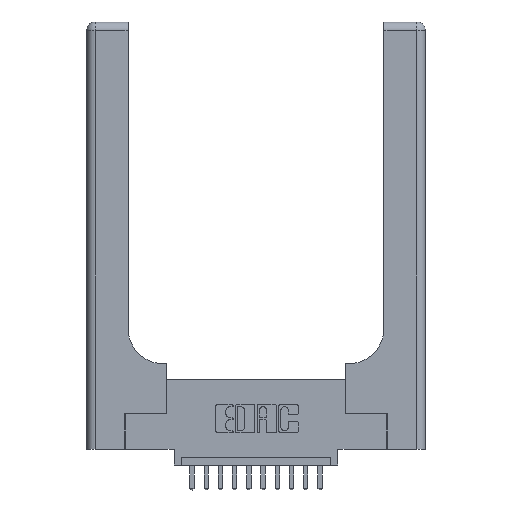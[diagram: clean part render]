
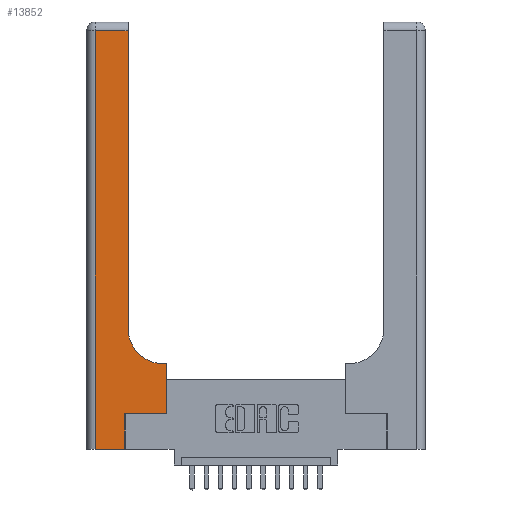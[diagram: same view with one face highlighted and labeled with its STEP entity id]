
A CAD part, top view. The second image highlights one B-rep face of the part: STEP entity #13852.
In plain terms, the highlighted planar face has unit normal (0, 0, 1).
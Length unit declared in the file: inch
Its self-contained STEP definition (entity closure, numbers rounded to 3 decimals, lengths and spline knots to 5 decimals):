
#390 = CARTESIAN_POINT ( 'NONE',  ( 0., 0., 0.37 ) ) ;
#481 = EDGE_CURVE ( 'NONE', #13509, #8513, #9069, .T. ) ;
#495 = CARTESIAN_POINT ( 'NONE',  ( 0.2915, 0.6, 0.37 ) ) ;
#685 = VERTEX_POINT ( 'NONE', #4158 ) ;
#1320 = DIRECTION ( 'NONE',  ( -1., 0., 0. ) ) ;
#1357 = CARTESIAN_POINT ( 'NONE',  ( 0.06, 0., 0.37 ) ) ;
#1411 = ORIENTED_EDGE ( 'NONE', *, *, #11169, .T. ) ;
#1579 = LINE ( 'NONE', #6632, #4900 ) ;
#1824 = ORIENTED_EDGE ( 'NONE', *, *, #481, .T. ) ;
#2064 = EDGE_CURVE ( 'NONE', #13979, #15824, #12297, .T. ) ;
#2503 = DIRECTION ( 'NONE',  ( 0., 1., 0. ) ) ;
#3252 = CARTESIAN_POINT ( 'NONE',  ( 0.269, 0.25, 0.37 ) ) ;
#3638 = LINE ( 'NONE', #14942, #13056 ) ;
#3772 = CARTESIAN_POINT ( 'NONE',  ( 0.2915, 3., 0.37 ) ) ;
#4047 = VERTEX_POINT ( 'NONE', #14977 ) ;
#4158 = CARTESIAN_POINT ( 'NONE',  ( 0.5585, 0.25, 0.37 ) ) ;
#4407 = EDGE_CURVE ( 'NONE', #7395, #13509, #3638, .T. ) ;
#4468 = VECTOR ( 'NONE', #13107, 39.37008 ) ;
#4494 = CIRCLE ( 'NONE', #12185, 0.25 ) ;
#4702 = CARTESIAN_POINT ( 'NONE',  ( 0.269, 0.25, 0.37 ) ) ;
#4900 = VECTOR ( 'NONE', #1320, 39.37008 ) ;
#5457 = EDGE_CURVE ( 'NONE', #685, #13979, #11946, .T. ) ;
#5551 = DIRECTION ( 'NONE',  ( 0., -1., 0. ) ) ;
#5587 = DIRECTION ( 'NONE',  ( 1., 0., 0. ) ) ;
#5896 = EDGE_CURVE ( 'NONE', #6042, #685, #9468, .T. ) ;
#6042 = VERTEX_POINT ( 'NONE', #3252 ) ;
#6632 = CARTESIAN_POINT ( 'NONE',  ( 0., 2.94, 0.37 ) ) ;
#7395 = VERTEX_POINT ( 'NONE', #13987 ) ;
#7418 = ORIENTED_EDGE ( 'NONE', *, *, #16864, .T. ) ;
#7435 = LINE ( 'NONE', #10268, #4468 ) ;
#7459 = CARTESIAN_POINT ( 'NONE',  ( 0.5415, 0.6, 0.37 ) ) ;
#8331 = DIRECTION ( 'NONE',  ( 1., 0., 0. ) ) ;
#8513 = VERTEX_POINT ( 'NONE', #10064 ) ;
#8906 = LINE ( 'NONE', #3772, #15551 ) ;
#9000 = EDGE_LOOP ( 'NONE', ( #7418, #13242, #15637, #1824, #1411, #16296, #9254, #10977, #16972 ) ) ;
#9045 = VECTOR ( 'NONE', #12773, 39.37008 ) ;
#9069 = LINE ( 'NONE', #390, #9901 ) ;
#9123 = DIRECTION ( 'NONE',  ( 0., 0., -1. ) ) ;
#9164 = DIRECTION ( 'NONE',  ( 0., 1., 0. ) ) ;
#9254 = ORIENTED_EDGE ( 'NONE', *, *, #5457, .T. ) ;
#9407 = CARTESIAN_POINT ( 'NONE',  ( 0.5585, 0.6, 0.37 ) ) ;
#9468 = LINE ( 'NONE', #4702, #9045 ) ;
#9586 = CARTESIAN_POINT ( 'NONE',  ( 0.5415, 0.85, 0.37 ) ) ;
#9901 = VECTOR ( 'NONE', #8331, 39.37008 ) ;
#10064 = CARTESIAN_POINT ( 'NONE',  ( 0.269, 0., 0.37 ) ) ;
#10241 = VECTOR ( 'NONE', #13913, 39.37008 ) ;
#10268 = CARTESIAN_POINT ( 'NONE',  ( 0.269, 0., 0.37 ) ) ;
#10322 = VECTOR ( 'NONE', #2503, 39.37008 ) ;
#10937 = AXIS2_PLACEMENT_3D ( 'NONE', #11952, #9123, #17013 ) ;
#10977 = ORIENTED_EDGE ( 'NONE', *, *, #2064, .T. ) ;
#11169 = EDGE_CURVE ( 'NONE', #8513, #6042, #7435, .T. ) ;
#11343 = EDGE_CURVE ( 'NONE', #4047, #7395, #1579, .T. ) ;
#11946 = LINE ( 'NONE', #15944, #10322 ) ;
#11952 = CARTESIAN_POINT ( 'NONE',  ( 0., 3., 0.37 ) ) ;
#12185 = AXIS2_PLACEMENT_3D ( 'NONE', #9586, #13364, #5587 ) ;
#12191 = CARTESIAN_POINT ( 'NONE',  ( 0.2915, 0.85, 0.37 ) ) ;
#12297 = LINE ( 'NONE', #495, #10241 ) ;
#12324 = FACE_OUTER_BOUND ( 'NONE', #9000, .T. ) ;
#12773 = DIRECTION ( 'NONE',  ( 1., 0., 0. ) ) ;
#13056 = VECTOR ( 'NONE', #5551, 39.37008 ) ;
#13107 = DIRECTION ( 'NONE',  ( 0., 1., 0. ) ) ;
#13242 = ORIENTED_EDGE ( 'NONE', *, *, #11343, .T. ) ;
#13364 = DIRECTION ( 'NONE',  ( 0., 0., -1. ) ) ;
#13509 = VERTEX_POINT ( 'NONE', #1357 ) ;
#13852 = ADVANCED_FACE ( 'NONE', ( #12324 ), #14646, .F. ) ;
#13913 = DIRECTION ( 'NONE',  ( -1., 0., 0. ) ) ;
#13979 = VERTEX_POINT ( 'NONE', #9407 ) ;
#13987 = CARTESIAN_POINT ( 'NONE',  ( 0.06, 2.94, 0.37 ) ) ;
#14646 = PLANE ( 'NONE',  #10937 ) ;
#14942 = CARTESIAN_POINT ( 'NONE',  ( 0.06, 3., 0.37 ) ) ;
#14977 = CARTESIAN_POINT ( 'NONE',  ( 0.2915, 2.94, 0.37 ) ) ;
#15079 = VERTEX_POINT ( 'NONE', #12191 ) ;
#15551 = VECTOR ( 'NONE', #9164, 39.37008 ) ;
#15637 = ORIENTED_EDGE ( 'NONE', *, *, #4407, .T. ) ;
#15824 = VERTEX_POINT ( 'NONE', #7459 ) ;
#15944 = CARTESIAN_POINT ( 'NONE',  ( 0.5585, 0.25, 0.37 ) ) ;
#16296 = ORIENTED_EDGE ( 'NONE', *, *, #5896, .T. ) ;
#16361 = EDGE_CURVE ( 'NONE', #15824, #15079, #4494, .T. ) ;
#16864 = EDGE_CURVE ( 'NONE', #15079, #4047, #8906, .T. ) ;
#16972 = ORIENTED_EDGE ( 'NONE', *, *, #16361, .T. ) ;
#17013 = DIRECTION ( 'NONE',  ( -1., 0., 0. ) ) ;
